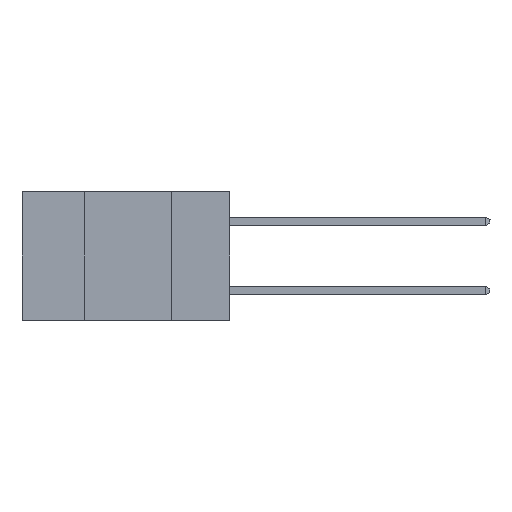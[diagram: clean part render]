
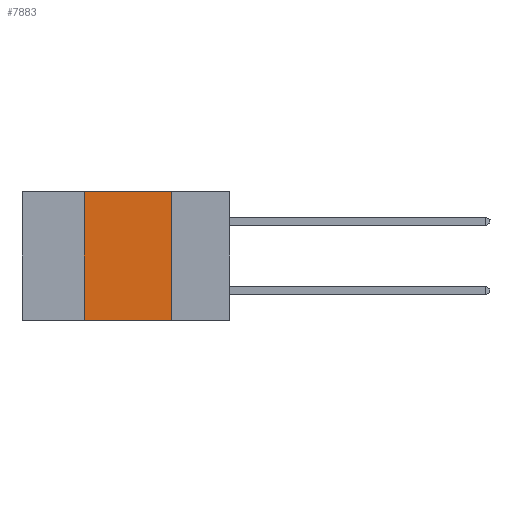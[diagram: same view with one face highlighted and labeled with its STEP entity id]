
A CAD part, left-side view. The second image highlights one B-rep face of the part: STEP entity #7883.
In plain terms, the highlighted planar face has unit normal (-1, 0, 0).
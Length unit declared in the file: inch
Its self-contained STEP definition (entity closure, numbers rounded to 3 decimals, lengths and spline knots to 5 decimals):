
#320 = ORIENTED_EDGE ( 'NONE', *, *, #997, .F. ) ;
#430 = DIRECTION ( 'NONE',  ( 0., 0., 1. ) ) ;
#997 = EDGE_CURVE ( 'NONE', #7230, #11247, #7867, .T. ) ;
#1227 = VECTOR ( 'NONE', #5590, 39.37008 ) ;
#1271 = DIRECTION ( 'NONE',  ( 0., 0., -1. ) ) ;
#1706 = ORIENTED_EDGE ( 'NONE', *, *, #13624, .F. ) ;
#1821 = VERTEX_POINT ( 'NONE', #9126 ) ;
#2463 = ORIENTED_EDGE ( 'NONE', *, *, #7159, .T. ) ;
#2532 = CARTESIAN_POINT ( 'NONE',  ( 0., 0.17, -0.37 ) ) ;
#2827 = EDGE_LOOP ( 'NONE', ( #320, #11933, #1706, #2463 ) ) ;
#5590 = DIRECTION ( 'NONE',  ( 0., -1., 0. ) ) ;
#5668 = LINE ( 'NONE', #13660, #7561 ) ;
#6071 = CARTESIAN_POINT ( 'NONE',  ( 0., 0.42, -0.37 ) ) ;
#6141 = CARTESIAN_POINT ( 'NONE',  ( 0., 0.6, 0. ) ) ;
#6583 = VECTOR ( 'NONE', #430, 39.37008 ) ;
#6808 = CARTESIAN_POINT ( 'NONE',  ( 0., 0.17, 0. ) ) ;
#7159 = EDGE_CURVE ( 'NONE', #1821, #11247, #5668, .T. ) ;
#7170 = LINE ( 'NONE', #6071, #6583 ) ;
#7230 = VERTEX_POINT ( 'NONE', #6808 ) ;
#7500 = CARTESIAN_POINT ( 'NONE',  ( 0., 0.42, 0. ) ) ;
#7561 = VECTOR ( 'NONE', #11173, 39.37008 ) ;
#7867 = LINE ( 'NONE', #2532, #9794 ) ;
#7883 = ADVANCED_FACE ( 'NONE', ( #10591 ), #8328, .F. ) ;
#8292 = VERTEX_POINT ( 'NONE', #7500 ) ;
#8328 = PLANE ( 'NONE',  #8384 ) ;
#8384 = AXIS2_PLACEMENT_3D ( 'NONE', #6141, #12774, #14010 ) ;
#9126 = CARTESIAN_POINT ( 'NONE',  ( 0., 0.42, -0.37 ) ) ;
#9794 = VECTOR ( 'NONE', #1271, 39.37008 ) ;
#10591 = FACE_OUTER_BOUND ( 'NONE', #2827, .T. ) ;
#11103 = CARTESIAN_POINT ( 'NONE',  ( 0., 0.6, 0. ) ) ;
#11173 = DIRECTION ( 'NONE',  ( 0., -1., 0. ) ) ;
#11247 = VERTEX_POINT ( 'NONE', #14326 ) ;
#11316 = LINE ( 'NONE', #11103, #1227 ) ;
#11420 = EDGE_CURVE ( 'NONE', #8292, #7230, #11316, .T. ) ;
#11933 = ORIENTED_EDGE ( 'NONE', *, *, #11420, .F. ) ;
#12774 = DIRECTION ( 'NONE',  ( 1., 0., 0. ) ) ;
#13624 = EDGE_CURVE ( 'NONE', #1821, #8292, #7170, .T. ) ;
#13660 = CARTESIAN_POINT ( 'NONE',  ( 0., 0.6, -0.37 ) ) ;
#14010 = DIRECTION ( 'NONE',  ( 0., 0., -1. ) ) ;
#14326 = CARTESIAN_POINT ( 'NONE',  ( 0., 0.17, -0.37 ) ) ;
